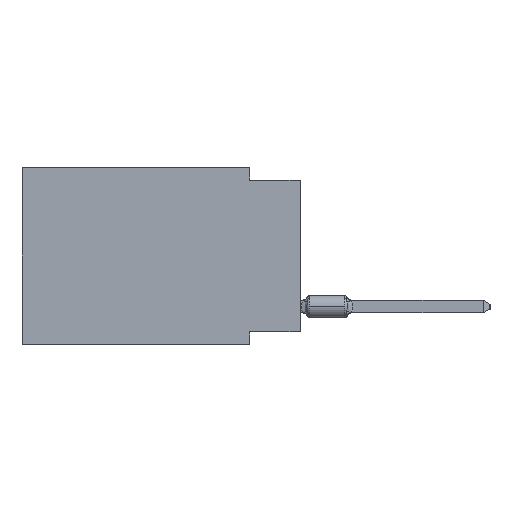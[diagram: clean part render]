
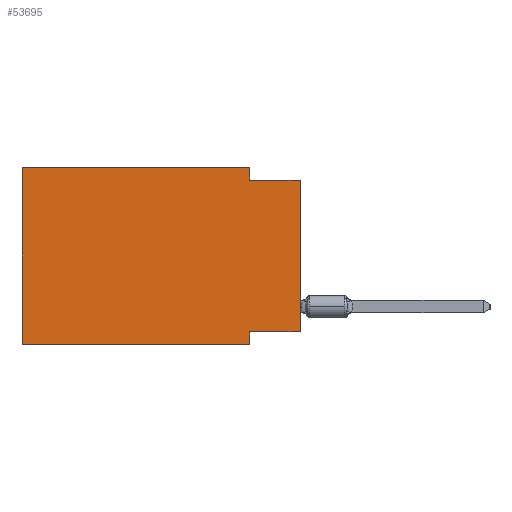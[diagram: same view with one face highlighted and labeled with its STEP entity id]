
A CAD part, left-side view. The second image highlights one B-rep face of the part: STEP entity #53695.
In plain terms, the highlighted planar face has unit normal (-1, 0, 0).
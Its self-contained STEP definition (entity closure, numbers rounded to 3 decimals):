
#410 = EDGE_LOOP ( 'NONE', ( #27239, #29429, #7411, #62287, #15484, #9988, #24324, #55254 ) ) ;
#685 = DIRECTION ( 'NONE',  ( 0., 0., -1. ) ) ;
#1162 = CARTESIAN_POINT ( 'NONE',  ( 0., 13.97, -8.89 ) ) ;
#1515 = VECTOR ( 'NONE', #50272, 1000. ) ;
#1733 = CARTESIAN_POINT ( 'NONE',  ( 0., 13.97, 0. ) ) ;
#2603 = LINE ( 'NONE', #7500, #19074 ) ;
#5334 = DIRECTION ( 'NONE',  ( 0., -1., 0. ) ) ;
#5609 = FACE_OUTER_BOUND ( 'NONE', #410, .T. ) ;
#7014 = VERTEX_POINT ( 'NONE', #53830 ) ;
#7411 = ORIENTED_EDGE ( 'NONE', *, *, #16363, .F. ) ;
#7500 = CARTESIAN_POINT ( 'NONE',  ( 0., 0., -0.635 ) ) ;
#7887 = CARTESIAN_POINT ( 'NONE',  ( 0., 0., -0.635 ) ) ;
#9988 = ORIENTED_EDGE ( 'NONE', *, *, #64135, .T. ) ;
#11497 = PLANE ( 'NONE',  #46860 ) ;
#14822 = CARTESIAN_POINT ( 'NONE',  ( 0., 2.54, -8.89 ) ) ;
#14918 = VECTOR ( 'NONE', #51389, 1000. ) ;
#15484 = ORIENTED_EDGE ( 'NONE', *, *, #64650, .F. ) ;
#15756 = VERTEX_POINT ( 'NONE', #7887 ) ;
#16363 = EDGE_CURVE ( 'NONE', #7014, #57297, #34601, .T. ) ;
#18290 = VECTOR ( 'NONE', #22356, 1000. ) ;
#19074 = VECTOR ( 'NONE', #47450, 1000. ) ;
#22356 = DIRECTION ( 'NONE',  ( 0., 0., 1. ) ) ;
#22896 = CARTESIAN_POINT ( 'NONE',  ( 0., 0., -8.255 ) ) ;
#23276 = VECTOR ( 'NONE', #35250, 1000. ) ;
#24137 = VECTOR ( 'NONE', #5334, 1000. ) ;
#24324 = ORIENTED_EDGE ( 'NONE', *, *, #28040, .F. ) ;
#25583 = CARTESIAN_POINT ( 'NONE',  ( 0., 13.97, 0. ) ) ;
#25708 = VERTEX_POINT ( 'NONE', #41914 ) ;
#27239 = ORIENTED_EDGE ( 'NONE', *, *, #54187, .T. ) ;
#27925 = CARTESIAN_POINT ( 'NONE',  ( 0., 2.54, -8.89 ) ) ;
#28040 = EDGE_CURVE ( 'NONE', #28618, #29565, #40682, .T. ) ;
#28618 = VERTEX_POINT ( 'NONE', #51962 ) ;
#29329 = LINE ( 'NONE', #43745, #46914 ) ;
#29429 = ORIENTED_EDGE ( 'NONE', *, *, #62348, .F. ) ;
#29565 = VERTEX_POINT ( 'NONE', #27925 ) ;
#30302 = LINE ( 'NONE', #1162, #1515 ) ;
#33454 = EDGE_CURVE ( 'NONE', #50981, #7014, #34488, .T. ) ;
#34168 = CARTESIAN_POINT ( 'NONE',  ( 0., 13.97, 0. ) ) ;
#34488 = LINE ( 'NONE', #34168, #24137 ) ;
#34601 = LINE ( 'NONE', #60151, #23276 ) ;
#35250 = DIRECTION ( 'NONE',  ( 0., 0., -1. ) ) ;
#40682 = LINE ( 'NONE', #14822, #62977 ) ;
#41914 = CARTESIAN_POINT ( 'NONE',  ( 0., 13.97, -8.89 ) ) ;
#43745 = CARTESIAN_POINT ( 'NONE',  ( 0., 0., 0. ) ) ;
#44570 = CARTESIAN_POINT ( 'NONE',  ( 0., 13.97, 0. ) ) ;
#45279 = DIRECTION ( 'NONE',  ( 0., 0., -1. ) ) ;
#45551 = DIRECTION ( 'NONE',  ( 1., 0., 0. ) ) ;
#46860 = AXIS2_PLACEMENT_3D ( 'NONE', #25583, #45551, #685 ) ;
#46914 = VECTOR ( 'NONE', #64383, 1000. ) ;
#47450 = DIRECTION ( 'NONE',  ( 0., -1., 0. ) ) ;
#47515 = CARTESIAN_POINT ( 'NONE',  ( 0., 2.54, -0.635 ) ) ;
#50272 = DIRECTION ( 'NONE',  ( 0., -1., 0. ) ) ;
#50981 = VERTEX_POINT ( 'NONE', #44570 ) ;
#51389 = DIRECTION ( 'NONE',  ( 0., 1., 0. ) ) ;
#51962 = CARTESIAN_POINT ( 'NONE',  ( 0., 2.54, -8.255 ) ) ;
#53695 = ADVANCED_FACE ( 'NONE', ( #5609 ), #11497, .F. ) ;
#53830 = CARTESIAN_POINT ( 'NONE',  ( 0., 2.54, 0. ) ) ;
#54187 = EDGE_CURVE ( 'NONE', #63116, #15756, #29329, .T. ) ;
#55254 = ORIENTED_EDGE ( 'NONE', *, *, #62350, .F. ) ;
#56091 = LINE ( 'NONE', #1733, #18290 ) ;
#57297 = VERTEX_POINT ( 'NONE', #47515 ) ;
#57924 = LINE ( 'NONE', #22896, #14918 ) ;
#59610 = CARTESIAN_POINT ( 'NONE',  ( 0., 0., -8.255 ) ) ;
#60151 = CARTESIAN_POINT ( 'NONE',  ( 0., 2.54, 0. ) ) ;
#62287 = ORIENTED_EDGE ( 'NONE', *, *, #33454, .F. ) ;
#62348 = EDGE_CURVE ( 'NONE', #57297, #15756, #2603, .T. ) ;
#62350 = EDGE_CURVE ( 'NONE', #63116, #28618, #57924, .T. ) ;
#62977 = VECTOR ( 'NONE', #45279, 1000. ) ;
#63116 = VERTEX_POINT ( 'NONE', #59610 ) ;
#64135 = EDGE_CURVE ( 'NONE', #25708, #29565, #30302, .T. ) ;
#64383 = DIRECTION ( 'NONE',  ( 0., 0., 1. ) ) ;
#64650 = EDGE_CURVE ( 'NONE', #25708, #50981, #56091, .T. ) ;
